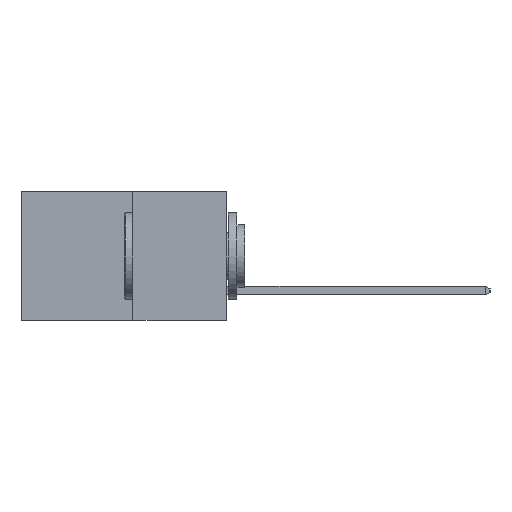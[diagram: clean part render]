
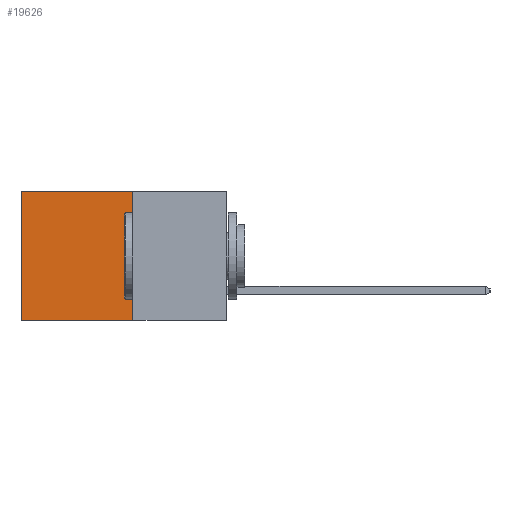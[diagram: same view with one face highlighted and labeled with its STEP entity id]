
A CAD part, left-side view. The second image highlights one B-rep face of the part: STEP entity #19626.
In plain terms, the highlighted planar face has unit normal (-1, 0, 0).
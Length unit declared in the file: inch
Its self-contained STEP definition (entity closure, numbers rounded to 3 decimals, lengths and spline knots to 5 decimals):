
#912 = PLANE ( 'NONE',  #18105 ) ;
#987 = DIRECTION ( 'NONE',  ( 0., 0., -1. ) ) ;
#2160 = VERTEX_POINT ( 'NONE', #20526 ) ;
#2973 = VERTEX_POINT ( 'NONE', #13267 ) ;
#3375 = DIRECTION ( 'NONE',  ( 0., 1., 0. ) ) ;
#4934 = DIRECTION ( 'NONE',  ( 1., 0., 0. ) ) ;
#5556 = LINE ( 'NONE', #17260, #15020 ) ;
#6758 = ORIENTED_EDGE ( 'NONE', *, *, #15827, .F. ) ;
#9030 = LINE ( 'NONE', #11532, #12487 ) ;
#9166 = DIRECTION ( 'NONE',  ( 0., 1., 0. ) ) ;
#10527 = VECTOR ( 'NONE', #3375, 39.37008 ) ;
#11532 = CARTESIAN_POINT ( 'NONE',  ( 0.277, 0.59, -0.37 ) ) ;
#12487 = VECTOR ( 'NONE', #23535, 39.37008 ) ;
#12547 = EDGE_CURVE ( 'NONE', #15683, #12929, #5556, .T. ) ;
#12654 = EDGE_CURVE ( 'NONE', #12929, #2160, #9030, .T. ) ;
#12929 = VERTEX_POINT ( 'NONE', #14435 ) ;
#13267 = CARTESIAN_POINT ( 'NONE',  ( 0.277, 0.27, -0.37 ) ) ;
#13768 = EDGE_LOOP ( 'NONE', ( #16282, #6758, #15198, #16627 ) ) ;
#14435 = CARTESIAN_POINT ( 'NONE',  ( 0.277, 0.59, 0. ) ) ;
#14976 = CARTESIAN_POINT ( 'NONE',  ( 0.277, 0.27, -0.37 ) ) ;
#15020 = VECTOR ( 'NONE', #9166, 39.37008 ) ;
#15198 = ORIENTED_EDGE ( 'NONE', *, *, #22937, .F. ) ;
#15246 = LINE ( 'NONE', #15535, #10527 ) ;
#15535 = CARTESIAN_POINT ( 'NONE',  ( 0.277, 0.27, -0.37 ) ) ;
#15683 = VERTEX_POINT ( 'NONE', #25074 ) ;
#15732 = LINE ( 'NONE', #16994, #20403 ) ;
#15827 = EDGE_CURVE ( 'NONE', #2973, #2160, #15246, .T. ) ;
#16282 = ORIENTED_EDGE ( 'NONE', *, *, #12654, .T. ) ;
#16627 = ORIENTED_EDGE ( 'NONE', *, *, #12547, .T. ) ;
#16994 = CARTESIAN_POINT ( 'NONE',  ( 0.277, 0.27, -0.37 ) ) ;
#17260 = CARTESIAN_POINT ( 'NONE',  ( 0.277, 0.27, 0. ) ) ;
#18105 = AXIS2_PLACEMENT_3D ( 'NONE', #14976, #4934, #18992 ) ;
#18992 = DIRECTION ( 'NONE',  ( 0., 0., -1. ) ) ;
#19626 = ADVANCED_FACE ( 'NONE', ( #21958 ), #912, .F. ) ;
#20403 = VECTOR ( 'NONE', #987, 39.37008 ) ;
#20526 = CARTESIAN_POINT ( 'NONE',  ( 0.277, 0.59, -0.37 ) ) ;
#21958 = FACE_OUTER_BOUND ( 'NONE', #13768, .T. ) ;
#22937 = EDGE_CURVE ( 'NONE', #15683, #2973, #15732, .T. ) ;
#23535 = DIRECTION ( 'NONE',  ( 0., 0., -1. ) ) ;
#25074 = CARTESIAN_POINT ( 'NONE',  ( 0.277, 0.27, 0. ) ) ;
